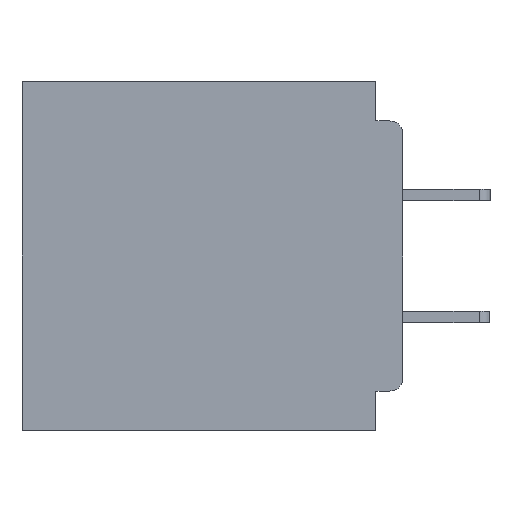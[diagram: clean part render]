
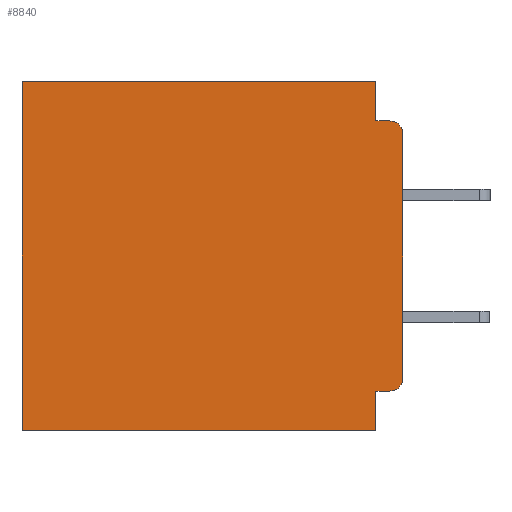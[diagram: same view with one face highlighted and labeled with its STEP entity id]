
A CAD part, left-side view. The second image highlights one B-rep face of the part: STEP entity #8840.
In plain terms, the highlighted planar face has unit normal (-1, 0, 0).
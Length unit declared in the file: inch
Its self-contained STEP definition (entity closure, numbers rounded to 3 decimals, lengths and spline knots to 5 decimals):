
#33 = LINE ( 'NONE', #25993, #20430 ) ;
#1190 = CARTESIAN_POINT ( 'NONE',  ( 0.3, 0.031, 0. ) ) ;
#1740 = CARTESIAN_POINT ( 'NONE',  ( 0.3, 0., -0.4 ) ) ;
#2139 = ORIENTED_EDGE ( 'NONE', *, *, #46013, .T. ) ;
#3694 = EDGE_LOOP ( 'NONE', ( #45610, #23550, #20918, #10743, #10037, #34679, #8761, #47539, #42107, #2139 ) ) ;
#5635 = DIRECTION ( 'NONE',  ( 0., 0., -1. ) ) ;
#5831 = CARTESIAN_POINT ( 'NONE',  ( 0.3, 0., -0.355 ) ) ;
#6686 = DIRECTION ( 'NONE',  ( -1., 0., 0. ) ) ;
#7373 = CARTESIAN_POINT ( 'NONE',  ( 0.3, 0.031, -0.355 ) ) ;
#8027 = PLANE ( 'NONE',  #50266 ) ;
#8761 = ORIENTED_EDGE ( 'NONE', *, *, #49583, .F. ) ;
#8840 = ADVANCED_FACE ( 'NONE', ( #30456 ), #8027, .F. ) ;
#9231 = CARTESIAN_POINT ( 'NONE',  ( 0.3, 0.437, -0.4 ) ) ;
#9876 = DIRECTION ( 'NONE',  ( 0., 1., 0. ) ) ;
#10037 = ORIENTED_EDGE ( 'NONE', *, *, #11379, .T. ) ;
#10225 = CARTESIAN_POINT ( 'NONE',  ( 0.3, 0., -0.34 ) ) ;
#10743 = ORIENTED_EDGE ( 'NONE', *, *, #42992, .F. ) ;
#10813 = VECTOR ( 'NONE', #25861, 39.37008 ) ;
#11040 = LINE ( 'NONE', #52088, #21930 ) ;
#11175 = VERTEX_POINT ( 'NONE', #34413 ) ;
#11379 = EDGE_CURVE ( 'NONE', #22275, #39656, #15553, .T. ) ;
#11774 = EDGE_CURVE ( 'NONE', #45364, #39453, #27677, .T. ) ;
#12134 = DIRECTION ( 'NONE',  ( 0., 0., -1. ) ) ;
#14523 = AXIS2_PLACEMENT_3D ( 'NONE', #31118, #6686, #35231 ) ;
#14854 = CARTESIAN_POINT ( 'NONE',  ( 0.3, 0.031, 0. ) ) ;
#15314 = CARTESIAN_POINT ( 'NONE',  ( 0.3, 0., 0. ) ) ;
#15553 = LINE ( 'NONE', #15314, #45459 ) ;
#15637 = DIRECTION ( 'NONE',  ( 0., 0., -1. ) ) ;
#16933 = LINE ( 'NONE', #1740, #48128 ) ;
#17613 = CARTESIAN_POINT ( 'NONE',  ( 0.3, 0., -0.045 ) ) ;
#19798 = EDGE_CURVE ( 'NONE', #39656, #28864, #40081, .T. ) ;
#20303 = CARTESIAN_POINT ( 'NONE',  ( 0.3, 0.015, -0.34 ) ) ;
#20430 = VECTOR ( 'NONE', #5635, 39.37008 ) ;
#20918 = ORIENTED_EDGE ( 'NONE', *, *, #32571, .F. ) ;
#21521 = DIRECTION ( 'NONE',  ( 0., 0., -1. ) ) ;
#21930 = VECTOR ( 'NONE', #15637, 39.37008 ) ;
#22257 = CARTESIAN_POINT ( 'NONE',  ( 0.3, 0.031, -0.045 ) ) ;
#22275 = VERTEX_POINT ( 'NONE', #14854 ) ;
#23550 = ORIENTED_EDGE ( 'NONE', *, *, #39312, .T. ) ;
#24410 = DIRECTION ( 'NONE',  ( 0., 0., -1. ) ) ;
#24439 = VERTEX_POINT ( 'NONE', #10225 ) ;
#25235 = CARTESIAN_POINT ( 'NONE',  ( 0.3, 0.437, 0. ) ) ;
#25712 = DIRECTION ( 'NONE',  ( 0., 0., -1. ) ) ;
#25729 = VECTOR ( 'NONE', #21521, 39.37008 ) ;
#25861 = DIRECTION ( 'NONE',  ( 0., -1., 0. ) ) ;
#25993 = CARTESIAN_POINT ( 'NONE',  ( 0.3, 0.031, -0.4 ) ) ;
#26206 = DIRECTION ( 'NONE',  ( 0., 1., 0. ) ) ;
#27677 = LINE ( 'NONE', #5831, #47970 ) ;
#28266 = LINE ( 'NONE', #1190, #25729 ) ;
#28329 = VERTEX_POINT ( 'NONE', #22257 ) ;
#28864 = VERTEX_POINT ( 'NONE', #29860 ) ;
#29512 = CARTESIAN_POINT ( 'NONE',  ( 0.3, 0.015, -0.045 ) ) ;
#29860 = CARTESIAN_POINT ( 'NONE',  ( 0.3, 0.437, -0.4 ) ) ;
#30456 = FACE_OUTER_BOUND ( 'NONE', #3694, .T. ) ;
#31118 = CARTESIAN_POINT ( 'NONE',  ( 0.3, 0.015, -0.06 ) ) ;
#31264 = VERTEX_POINT ( 'NONE', #34273 ) ;
#31311 = CIRCLE ( 'NONE', #37875, 0.015 ) ;
#31729 = DIRECTION ( 'NONE',  ( 0., 1., 0. ) ) ;
#32495 = CARTESIAN_POINT ( 'NONE',  ( 0.3, 0., -0.4 ) ) ;
#32571 = EDGE_CURVE ( 'NONE', #28329, #41693, #43316, .T. ) ;
#34273 = CARTESIAN_POINT ( 'NONE',  ( 0.3, 0.031, -0.4 ) ) ;
#34413 = CARTESIAN_POINT ( 'NONE',  ( 0.3, 0., -0.06 ) ) ;
#34679 = ORIENTED_EDGE ( 'NONE', *, *, #19798, .T. ) ;
#35231 = DIRECTION ( 'NONE',  ( 0., 0., -1. ) ) ;
#36559 = DIRECTION ( 'NONE',  ( 1., 0., 0. ) ) ;
#37875 = AXIS2_PLACEMENT_3D ( 'NONE', #20303, #48748, #24410 ) ;
#38821 = VECTOR ( 'NONE', #25712, 39.37008 ) ;
#39312 = EDGE_CURVE ( 'NONE', #11175, #41693, #41984, .T. ) ;
#39453 = VERTEX_POINT ( 'NONE', #7373 ) ;
#39656 = VERTEX_POINT ( 'NONE', #25235 ) ;
#40081 = LINE ( 'NONE', #9231, #38821 ) ;
#40429 = CARTESIAN_POINT ( 'NONE',  ( 0.3, 0.015, -0.355 ) ) ;
#41693 = VERTEX_POINT ( 'NONE', #29512 ) ;
#41984 = CIRCLE ( 'NONE', #14523, 0.015 ) ;
#42107 = ORIENTED_EDGE ( 'NONE', *, *, #11774, .F. ) ;
#42992 = EDGE_CURVE ( 'NONE', #22275, #28329, #28266, .T. ) ;
#43316 = LINE ( 'NONE', #17613, #10813 ) ;
#44448 = EDGE_CURVE ( 'NONE', #39453, #31264, #33, .T. ) ;
#45364 = VERTEX_POINT ( 'NONE', #40429 ) ;
#45459 = VECTOR ( 'NONE', #31729, 39.37008 ) ;
#45610 = ORIENTED_EDGE ( 'NONE', *, *, #52111, .F. ) ;
#46013 = EDGE_CURVE ( 'NONE', #45364, #24439, #31311, .T. ) ;
#47539 = ORIENTED_EDGE ( 'NONE', *, *, #44448, .F. ) ;
#47970 = VECTOR ( 'NONE', #9876, 39.37008 ) ;
#48128 = VECTOR ( 'NONE', #26206, 39.37008 ) ;
#48748 = DIRECTION ( 'NONE',  ( -1., 0., 0. ) ) ;
#49583 = EDGE_CURVE ( 'NONE', #31264, #28864, #16933, .T. ) ;
#50266 = AXIS2_PLACEMENT_3D ( 'NONE', #32495, #36559, #12134 ) ;
#52088 = CARTESIAN_POINT ( 'NONE',  ( 0.3, 0., -0.4 ) ) ;
#52111 = EDGE_CURVE ( 'NONE', #11175, #24439, #11040, .T. ) ;
